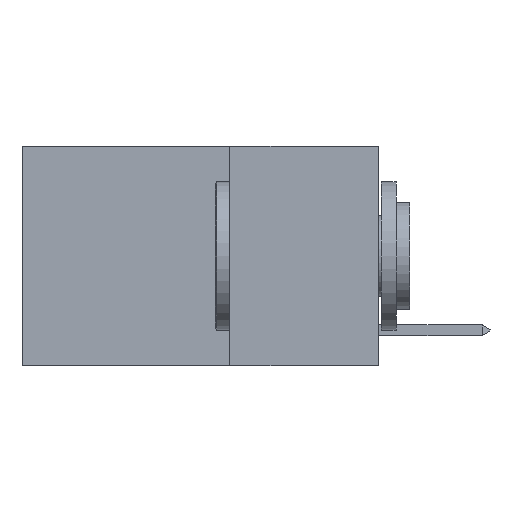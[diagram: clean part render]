
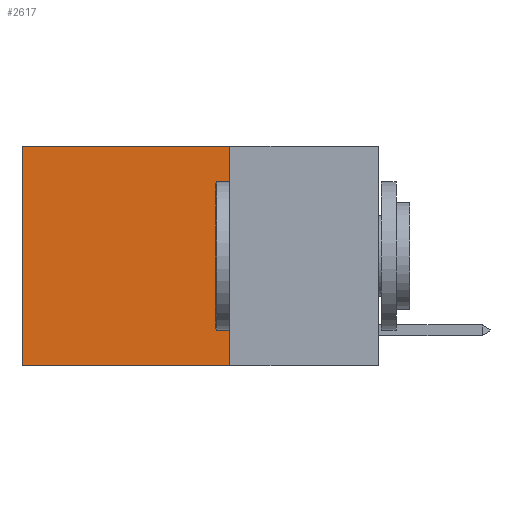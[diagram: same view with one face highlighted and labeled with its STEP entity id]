
A CAD part, left-side view. The second image highlights one B-rep face of the part: STEP entity #2617.
In plain terms, the highlighted planar face has unit normal (-1, 0, 0).
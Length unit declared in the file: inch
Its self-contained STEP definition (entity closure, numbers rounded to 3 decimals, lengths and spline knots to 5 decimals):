
#559 = VECTOR ( 'NONE', #17635, 39.37008 ) ;
#1030 = LINE ( 'NONE', #17349, #559 ) ;
#1792 = EDGE_CURVE ( 'NONE', #13539, #4559, #11208, .T. ) ;
#2379 = EDGE_CURVE ( 'NONE', #13539, #3487, #1030, .T. ) ;
#2508 = CARTESIAN_POINT ( 'NONE',  ( 0.2625, 0.25, 0. ) ) ;
#2617 = ADVANCED_FACE ( 'NONE', ( #17615 ), #17784, .F. ) ;
#2639 = VECTOR ( 'NONE', #3194, 39.37008 ) ;
#3194 = DIRECTION ( 'NONE',  ( 0., 1., 0. ) ) ;
#3266 = DIRECTION ( 'NONE',  ( 0., 0., -1. ) ) ;
#3487 = VERTEX_POINT ( 'NONE', #5742 ) ;
#3648 = CARTESIAN_POINT ( 'NONE',  ( 0.2625, 0.25, -0.37 ) ) ;
#3662 = EDGE_CURVE ( 'NONE', #4559, #18152, #14162, .T. ) ;
#4559 = VERTEX_POINT ( 'NONE', #4752 ) ;
#4752 = CARTESIAN_POINT ( 'NONE',  ( 0.2625, 0.25, -0.37 ) ) ;
#4893 = CARTESIAN_POINT ( 'NONE',  ( 0.2625, 0.6, 0. ) ) ;
#5677 = LINE ( 'NONE', #4893, #17312 ) ;
#5742 = CARTESIAN_POINT ( 'NONE',  ( 0.2625, 0.6, 0. ) ) ;
#5932 = ORIENTED_EDGE ( 'NONE', *, *, #15456, .T. ) ;
#6000 = ORIENTED_EDGE ( 'NONE', *, *, #3662, .F. ) ;
#6141 = ORIENTED_EDGE ( 'NONE', *, *, #1792, .F. ) ;
#6256 = ORIENTED_EDGE ( 'NONE', *, *, #2379, .T. ) ;
#7449 = VECTOR ( 'NONE', #3266, 39.37008 ) ;
#8351 = AXIS2_PLACEMENT_3D ( 'NONE', #17731, #17713, #17699 ) ;
#11208 = LINE ( 'NONE', #2508, #7449 ) ;
#13539 = VERTEX_POINT ( 'NONE', #14836 ) ;
#14162 = LINE ( 'NONE', #3648, #2639 ) ;
#14650 = CARTESIAN_POINT ( 'NONE',  ( 0.2625, 0.6, -0.37 ) ) ;
#14798 = DIRECTION ( 'NONE',  ( 0., 0., -1. ) ) ;
#14836 = CARTESIAN_POINT ( 'NONE',  ( 0.2625, 0.25, 0. ) ) ;
#15456 = EDGE_CURVE ( 'NONE', #3487, #18152, #5677, .T. ) ;
#17250 = EDGE_LOOP ( 'NONE', ( #5932, #6000, #6141, #6256 ) ) ;
#17312 = VECTOR ( 'NONE', #14798, 39.37008 ) ;
#17349 = CARTESIAN_POINT ( 'NONE',  ( 0.2625, 0.25, 0. ) ) ;
#17615 = FACE_OUTER_BOUND ( 'NONE', #17250, .T. ) ;
#17635 = DIRECTION ( 'NONE',  ( 0., 1., 0. ) ) ;
#17699 = DIRECTION ( 'NONE',  ( 0., 0., -1. ) ) ;
#17713 = DIRECTION ( 'NONE',  ( 1., 0., 0. ) ) ;
#17731 = CARTESIAN_POINT ( 'NONE',  ( 0.2625, 0.25, 0. ) ) ;
#17784 = PLANE ( 'NONE',  #8351 ) ;
#18152 = VERTEX_POINT ( 'NONE', #14650 ) ;
